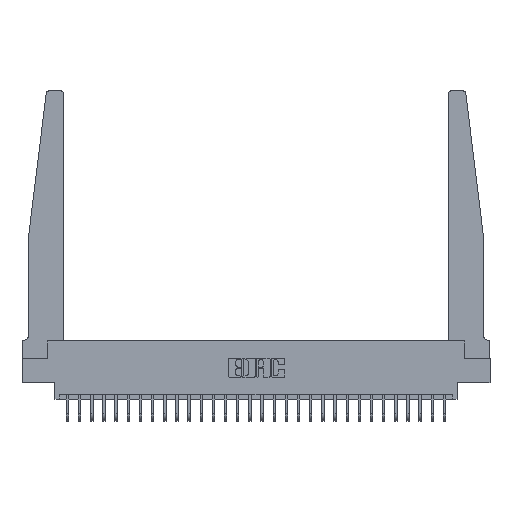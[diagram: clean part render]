
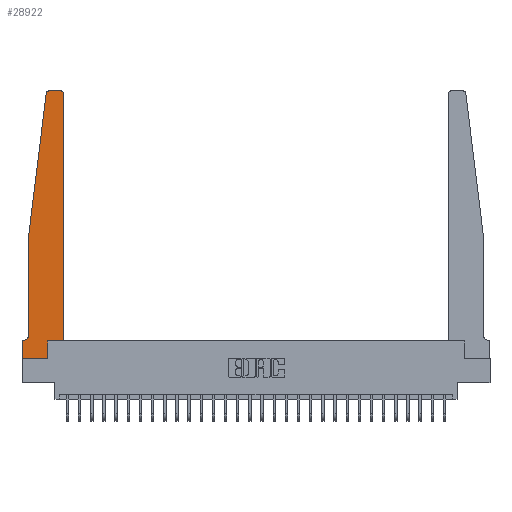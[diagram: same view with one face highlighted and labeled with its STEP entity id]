
A CAD part, top view. The second image highlights one B-rep face of the part: STEP entity #28922.
In plain terms, the highlighted planar face has unit normal (0, 0, 1).
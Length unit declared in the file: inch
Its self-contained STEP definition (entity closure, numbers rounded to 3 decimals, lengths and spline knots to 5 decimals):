
#382 = LINE ( 'NONE', #25510, #8149 ) ;
#403 = ORIENTED_EDGE ( 'NONE', *, *, #8215, .T. ) ;
#630 = CARTESIAN_POINT ( 'NONE',  ( 0.27653, 2.75, 0.37 ) ) ;
#905 = ORIENTED_EDGE ( 'NONE', *, *, #5936, .T. ) ;
#1336 = DIRECTION ( 'NONE',  ( 0., -1., 0. ) ) ;
#1386 = CIRCLE ( 'NONE', #20878, 0.03 ) ;
#1613 = CARTESIAN_POINT ( 'NONE',  ( 0.24675, 2.72367, 0.37 ) ) ;
#1898 = CARTESIAN_POINT ( 'NONE',  ( 0.425, 0.18, 0.37 ) ) ;
#2368 = DIRECTION ( 'NONE',  ( 0., 0., 1. ) ) ;
#2670 = AXIS2_PLACEMENT_3D ( 'NONE', #10821, #26401, #6054 ) ;
#2717 = VERTEX_POINT ( 'NONE', #27213 ) ;
#3231 = ORIENTED_EDGE ( 'NONE', *, *, #12702, .T. ) ;
#3743 = CARTESIAN_POINT ( 'NONE',  ( 0.425, 2.72, 0.37 ) ) ;
#3864 = VERTEX_POINT ( 'NONE', #16670 ) ;
#4195 = VERTEX_POINT ( 'NONE', #10663 ) ;
#4685 = DIRECTION ( 'NONE',  ( 0., 1., 0. ) ) ;
#5078 = VERTEX_POINT ( 'NONE', #19278 ) ;
#5368 = EDGE_CURVE ( 'NONE', #5078, #5650, #25049, .T. ) ;
#5404 = LINE ( 'NONE', #12407, #24843 ) ;
#5465 = CARTESIAN_POINT ( 'NONE',  ( 0.425, 0.18, 0.37 ) ) ;
#5497 = VERTEX_POINT ( 'NONE', #5986 ) ;
#5518 = VERTEX_POINT ( 'NONE', #3743 ) ;
#5650 = VERTEX_POINT ( 'NONE', #630 ) ;
#5788 = DIRECTION ( 'NONE',  ( 0., 0., 1. ) ) ;
#5910 = DIRECTION ( 'NONE',  ( 1., 0., 0. ) ) ;
#5936 = EDGE_CURVE ( 'NONE', #29109, #5518, #9540, .T. ) ;
#5986 = CARTESIAN_POINT ( 'NONE',  ( 0.2605, 0.18, 0.37 ) ) ;
#6054 = DIRECTION ( 'NONE',  ( -1., 0., 0. ) ) ;
#6555 = CIRCLE ( 'NONE', #11799, 0.03 ) ;
#6912 = CARTESIAN_POINT ( 'NONE',  ( 0.25, 2.75, 0.37 ) ) ;
#7152 = VERTEX_POINT ( 'NONE', #12656 ) ;
#8067 = LINE ( 'NONE', #24235, #10842 ) ;
#8096 = LINE ( 'NONE', #21744, #13640 ) ;
#8149 = VECTOR ( 'NONE', #25667, 39.37008 ) ;
#8215 = EDGE_CURVE ( 'NONE', #2717, #5497, #18518, .T. ) ;
#8327 = CARTESIAN_POINT ( 'NONE',  ( 0.27653, 2.72, 0.37 ) ) ;
#9411 = ORIENTED_EDGE ( 'NONE', *, *, #24950, .T. ) ;
#9540 = LINE ( 'NONE', #23182, #15676 ) ;
#9870 = ORIENTED_EDGE ( 'NONE', *, *, #18694, .T. ) ;
#10091 = LINE ( 'NONE', #5465, #28765 ) ;
#10663 = CARTESIAN_POINT ( 'NONE',  ( 0.015, 0.1875, 0.37 ) ) ;
#10821 = CARTESIAN_POINT ( 'NONE',  ( 0.015, 0.2375, 0.37 ) ) ;
#10842 = VECTOR ( 'NONE', #1336, 39.37008 ) ;
#11038 = ORIENTED_EDGE ( 'NONE', *, *, #14485, .T. ) ;
#11606 = ORIENTED_EDGE ( 'NONE', *, *, #25764, .T. ) ;
#11616 = DIRECTION ( 'NONE',  ( 0., 1., 0. ) ) ;
#11799 = AXIS2_PLACEMENT_3D ( 'NONE', #14991, #26408, #5910 ) ;
#12162 = VECTOR ( 'NONE', #15373, 39.37008 ) ;
#12407 = CARTESIAN_POINT ( 'NONE',  ( 0., 0., 0.37 ) ) ;
#12544 = DIRECTION ( 'NONE',  ( -0.122, -0.992, 0. ) ) ;
#12656 = CARTESIAN_POINT ( 'NONE',  ( 0., 0.1875, 0.37 ) ) ;
#12702 = EDGE_CURVE ( 'NONE', #7152, #16572, #382, .T. ) ;
#12845 = CARTESIAN_POINT ( 'NONE',  ( 0.065, 0.2375, 0.37 ) ) ;
#13640 = VECTOR ( 'NONE', #12544, 39.37008 ) ;
#14485 = EDGE_CURVE ( 'NONE', #19941, #3864, #8096, .T. ) ;
#14806 = CARTESIAN_POINT ( 'NONE',  ( 0., 0., 0.37 ) ) ;
#14860 = DIRECTION ( 'NONE',  ( 1., 0., 0. ) ) ;
#14991 = CARTESIAN_POINT ( 'NONE',  ( 0.395, 2.72, 0.37 ) ) ;
#15358 = EDGE_CURVE ( 'NONE', #5518, #5078, #6555, .T. ) ;
#15373 = DIRECTION ( 'NONE',  ( -1., 0., 0. ) ) ;
#15676 = VECTOR ( 'NONE', #11616, 39.37008 ) ;
#15692 = EDGE_LOOP ( 'NONE', ( #20046, #18265, #11038, #9870, #25299, #9411, #3231, #15940, #403, #11606, #905, #15832 ) ) ;
#15832 = ORIENTED_EDGE ( 'NONE', *, *, #15358, .T. ) ;
#15940 = ORIENTED_EDGE ( 'NONE', *, *, #21258, .T. ) ;
#15987 = DIRECTION ( 'NONE',  ( -1., 0., 0. ) ) ;
#16104 = AXIS2_PLACEMENT_3D ( 'NONE', #22745, #2368, #20537 ) ;
#16223 = EDGE_CURVE ( 'NONE', #17038, #4195, #21222, .T. ) ;
#16572 = VERTEX_POINT ( 'NONE', #14806 ) ;
#16670 = CARTESIAN_POINT ( 'NONE',  ( 0.065, 1.25, 0.37 ) ) ;
#16774 = DIRECTION ( 'NONE',  ( 1., 0., 0. ) ) ;
#17038 = VERTEX_POINT ( 'NONE', #12845 ) ;
#18265 = ORIENTED_EDGE ( 'NONE', *, *, #29197, .T. ) ;
#18518 = LINE ( 'NONE', #20457, #23252 ) ;
#18575 = VECTOR ( 'NONE', #15987, 39.37008 ) ;
#18694 = EDGE_CURVE ( 'NONE', #3864, #17038, #8067, .T. ) ;
#19278 = CARTESIAN_POINT ( 'NONE',  ( 0.395, 2.75, 0.37 ) ) ;
#19941 = VERTEX_POINT ( 'NONE', #1613 ) ;
#20046 = ORIENTED_EDGE ( 'NONE', *, *, #5368, .T. ) ;
#20231 = PLANE ( 'NONE',  #16104 ) ;
#20457 = CARTESIAN_POINT ( 'NONE',  ( 0.2605, 0.18, 0.37 ) ) ;
#20537 = DIRECTION ( 'NONE',  ( 1., 0., 0. ) ) ;
#20878 = AXIS2_PLACEMENT_3D ( 'NONE', #8327, #5788, #14860 ) ;
#21222 = CIRCLE ( 'NONE', #2670, 0.05 ) ;
#21258 = EDGE_CURVE ( 'NONE', #16572, #2717, #5404, .T. ) ;
#21744 = CARTESIAN_POINT ( 'NONE',  ( 0.065, 1.25, 0.37 ) ) ;
#22745 = CARTESIAN_POINT ( 'NONE',  ( 0., 0.1875, 0.37 ) ) ;
#23182 = CARTESIAN_POINT ( 'NONE',  ( 0.425, 0.18, 0.37 ) ) ;
#23252 = VECTOR ( 'NONE', #4685, 39.37008 ) ;
#24235 = CARTESIAN_POINT ( 'NONE',  ( 0.065, 1.25, 0.37 ) ) ;
#24281 = CARTESIAN_POINT ( 'NONE',  ( 0.065, 0.1875, 0.37 ) ) ;
#24843 = VECTOR ( 'NONE', #27992, 39.37008 ) ;
#24950 = EDGE_CURVE ( 'NONE', #4195, #7152, #29024, .T. ) ;
#25049 = LINE ( 'NONE', #6912, #18575 ) ;
#25299 = ORIENTED_EDGE ( 'NONE', *, *, #16223, .T. ) ;
#25510 = CARTESIAN_POINT ( 'NONE',  ( 0., 0., 0.37 ) ) ;
#25667 = DIRECTION ( 'NONE',  ( 0., -1., 0. ) ) ;
#25764 = EDGE_CURVE ( 'NONE', #5497, #29109, #10091, .T. ) ;
#26401 = DIRECTION ( 'NONE',  ( 0., 0., -1. ) ) ;
#26408 = DIRECTION ( 'NONE',  ( 0., 0., 1. ) ) ;
#27213 = CARTESIAN_POINT ( 'NONE',  ( 0.2605, 0., 0.37 ) ) ;
#27992 = DIRECTION ( 'NONE',  ( 1., 0., 0. ) ) ;
#28765 = VECTOR ( 'NONE', #16774, 39.37008 ) ;
#28922 = ADVANCED_FACE ( 'NONE', ( #29278 ), #20231, .T. ) ;
#29024 = LINE ( 'NONE', #24281, #12162 ) ;
#29109 = VERTEX_POINT ( 'NONE', #1898 ) ;
#29197 = EDGE_CURVE ( 'NONE', #5650, #19941, #1386, .T. ) ;
#29278 = FACE_OUTER_BOUND ( 'NONE', #15692, .T. ) ;
